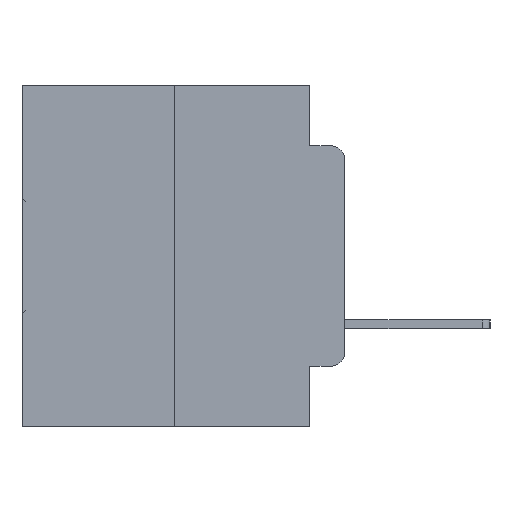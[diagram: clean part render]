
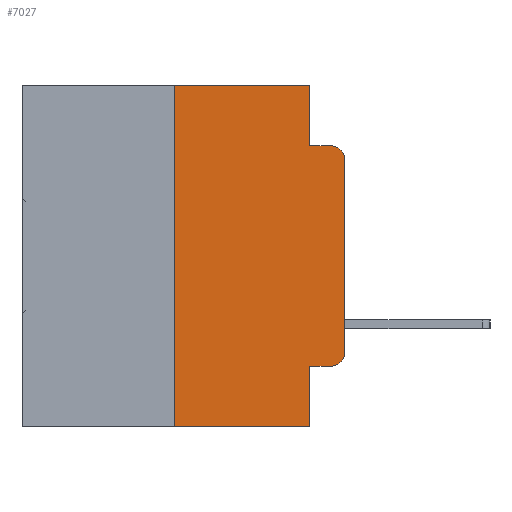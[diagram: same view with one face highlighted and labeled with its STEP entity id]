
A CAD part, left-side view. The second image highlights one B-rep face of the part: STEP entity #7027.
In plain terms, the highlighted planar face has unit normal (-1, 0, 0).
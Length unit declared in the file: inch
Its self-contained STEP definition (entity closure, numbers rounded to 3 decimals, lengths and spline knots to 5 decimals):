
#717 = DIRECTION ( 'NONE',  ( -1., 0., 0. ) ) ;
#726 = DIRECTION ( 'NONE',  ( 0., -1., 0. ) ) ;
#906 = ORIENTED_EDGE ( 'NONE', *, *, #27805, .T. ) ;
#1099 = VERTEX_POINT ( 'NONE', #27862 ) ;
#1607 = CARTESIAN_POINT ( 'NONE',  ( 0., 0.051, 0. ) ) ;
#2036 = AXIS2_PLACEMENT_3D ( 'NONE', #15566, #717, #18018 ) ;
#2437 = VERTEX_POINT ( 'NONE', #18723 ) ;
#2552 = VECTOR ( 'NONE', #726, 39.37008 ) ;
#2983 = ORIENTED_EDGE ( 'NONE', *, *, #28405, .F. ) ;
#3188 = DIRECTION ( 'NONE',  ( 0., 0., -1. ) ) ;
#3299 = DIRECTION ( 'NONE',  ( 0., -1., 0. ) ) ;
#3764 = CARTESIAN_POINT ( 'NONE',  ( 0., 0.051, -0.0885 ) ) ;
#3809 = VERTEX_POINT ( 'NONE', #11767 ) ;
#4159 = CIRCLE ( 'NONE', #7585, 0.02 ) ;
#4473 = ORIENTED_EDGE ( 'NONE', *, *, #25746, .T. ) ;
#4571 = VECTOR ( 'NONE', #7291, 39.37008 ) ;
#4629 = LINE ( 'NONE', #10220, #16225 ) ;
#5188 = VERTEX_POINT ( 'NONE', #31771 ) ;
#5405 = VERTEX_POINT ( 'NONE', #22820 ) ;
#5565 = CARTESIAN_POINT ( 'NONE',  ( 0., 0.25, 0. ) ) ;
#5988 = EDGE_CURVE ( 'NONE', #1099, #2437, #15559, .T. ) ;
#6580 = DIRECTION ( 'NONE',  ( 0., 0., -1. ) ) ;
#7027 = ADVANCED_FACE ( 'NONE', ( #16614 ), #22759, .F. ) ;
#7291 = DIRECTION ( 'NONE',  ( 0., -1., 0. ) ) ;
#7353 = CARTESIAN_POINT ( 'NONE',  ( 0., 0.25, 0. ) ) ;
#7585 = AXIS2_PLACEMENT_3D ( 'NONE', #10692, #27824, #13206 ) ;
#7935 = DIRECTION ( 'NONE',  ( 0., 0., 1. ) ) ;
#8440 = ORIENTED_EDGE ( 'NONE', *, *, #21856, .F. ) ;
#9803 = CARTESIAN_POINT ( 'NONE',  ( 0., 0.473, -0.5 ) ) ;
#9914 = LINE ( 'NONE', #30147, #2552 ) ;
#10220 = CARTESIAN_POINT ( 'NONE',  ( 0., 0.051, 0. ) ) ;
#10692 = CARTESIAN_POINT ( 'NONE',  ( 0., 0.02, -0.1085 ) ) ;
#11767 = CARTESIAN_POINT ( 'NONE',  ( 0., 0., -0.1085 ) ) ;
#12812 = VECTOR ( 'NONE', #6580, 39.37008 ) ;
#13092 = CARTESIAN_POINT ( 'NONE',  ( 0., 0., 0. ) ) ;
#13206 = DIRECTION ( 'NONE',  ( 0., 0., -1. ) ) ;
#13686 = EDGE_CURVE ( 'NONE', #23154, #22943, #19330, .T. ) ;
#14741 = EDGE_CURVE ( 'NONE', #17619, #18588, #16983, .T. ) ;
#15129 = LINE ( 'NONE', #13092, #28097 ) ;
#15262 = ORIENTED_EDGE ( 'NONE', *, *, #21234, .T. ) ;
#15559 = CIRCLE ( 'NONE', #2036, 0.02 ) ;
#15566 = CARTESIAN_POINT ( 'NONE',  ( 0., 0.02, -0.3915 ) ) ;
#15649 = EDGE_CURVE ( 'NONE', #16765, #5188, #9914, .T. ) ;
#16225 = VECTOR ( 'NONE', #20102, 39.37008 ) ;
#16614 = FACE_OUTER_BOUND ( 'NONE', #27333, .T. ) ;
#16765 = VERTEX_POINT ( 'NONE', #7353 ) ;
#16983 = LINE ( 'NONE', #18098, #20391 ) ;
#17191 = VECTOR ( 'NONE', #19333, 39.37008 ) ;
#17619 = VERTEX_POINT ( 'NONE', #3764 ) ;
#17998 = DIRECTION ( 'NONE',  ( 1., 0., 0. ) ) ;
#18018 = DIRECTION ( 'NONE',  ( 0., 0., -1. ) ) ;
#18098 = CARTESIAN_POINT ( 'NONE',  ( 0., 0.051, -0.0885 ) ) ;
#18336 = ORIENTED_EDGE ( 'NONE', *, *, #14741, .F. ) ;
#18412 = ORIENTED_EDGE ( 'NONE', *, *, #13686, .F. ) ;
#18588 = VERTEX_POINT ( 'NONE', #29020 ) ;
#18723 = CARTESIAN_POINT ( 'NONE',  ( 0., 0., -0.3915 ) ) ;
#18755 = ORIENTED_EDGE ( 'NONE', *, *, #5988, .T. ) ;
#19330 = LINE ( 'NONE', #1607, #12812 ) ;
#19333 = DIRECTION ( 'NONE',  ( 0., -1., 0. ) ) ;
#20102 = DIRECTION ( 'NONE',  ( 0., 0., -1. ) ) ;
#20391 = VECTOR ( 'NONE', #3299, 39.37008 ) ;
#21138 = ORIENTED_EDGE ( 'NONE', *, *, #21666, .T. ) ;
#21234 = EDGE_CURVE ( 'NONE', #3809, #18588, #4159, .T. ) ;
#21666 = EDGE_CURVE ( 'NONE', #5405, #22943, #23735, .T. ) ;
#21856 = EDGE_CURVE ( 'NONE', #5405, #16765, #25312, .T. ) ;
#21879 = ORIENTED_EDGE ( 'NONE', *, *, #15649, .F. ) ;
#22759 = PLANE ( 'NONE',  #26576 ) ;
#22820 = CARTESIAN_POINT ( 'NONE',  ( 0., 0.25, -0.5 ) ) ;
#22943 = VERTEX_POINT ( 'NONE', #31734 ) ;
#23154 = VERTEX_POINT ( 'NONE', #30253 ) ;
#23735 = LINE ( 'NONE', #9803, #4571 ) ;
#25312 = LINE ( 'NONE', #5565, #30999 ) ;
#25746 = EDGE_CURVE ( 'NONE', #23154, #1099, #30132, .T. ) ;
#26576 = AXIS2_PLACEMENT_3D ( 'NONE', #30117, #17998, #3188 ) ;
#27333 = EDGE_LOOP ( 'NONE', ( #906, #15262, #18336, #2983, #21879, #8440, #21138, #18412, #4473, #18755 ) ) ;
#27805 = EDGE_CURVE ( 'NONE', #2437, #3809, #15129, .T. ) ;
#27824 = DIRECTION ( 'NONE',  ( -1., 0., 0. ) ) ;
#27862 = CARTESIAN_POINT ( 'NONE',  ( 0., 0.02, -0.4115 ) ) ;
#28097 = VECTOR ( 'NONE', #30156, 39.37008 ) ;
#28405 = EDGE_CURVE ( 'NONE', #5188, #17619, #4629, .T. ) ;
#29020 = CARTESIAN_POINT ( 'NONE',  ( 0., 0.02, -0.0885 ) ) ;
#29024 = CARTESIAN_POINT ( 'NONE',  ( 0., 0.051, -0.4115 ) ) ;
#30117 = CARTESIAN_POINT ( 'NONE',  ( 0., 0.473, 0. ) ) ;
#30132 = LINE ( 'NONE', #29024, #17191 ) ;
#30147 = CARTESIAN_POINT ( 'NONE',  ( 0., 0.473, 0. ) ) ;
#30156 = DIRECTION ( 'NONE',  ( 0., 0., 1. ) ) ;
#30253 = CARTESIAN_POINT ( 'NONE',  ( 0., 0.051, -0.4115 ) ) ;
#30999 = VECTOR ( 'NONE', #7935, 39.37008 ) ;
#31734 = CARTESIAN_POINT ( 'NONE',  ( 0., 0.051, -0.5 ) ) ;
#31771 = CARTESIAN_POINT ( 'NONE',  ( 0., 0.051, 0. ) ) ;
